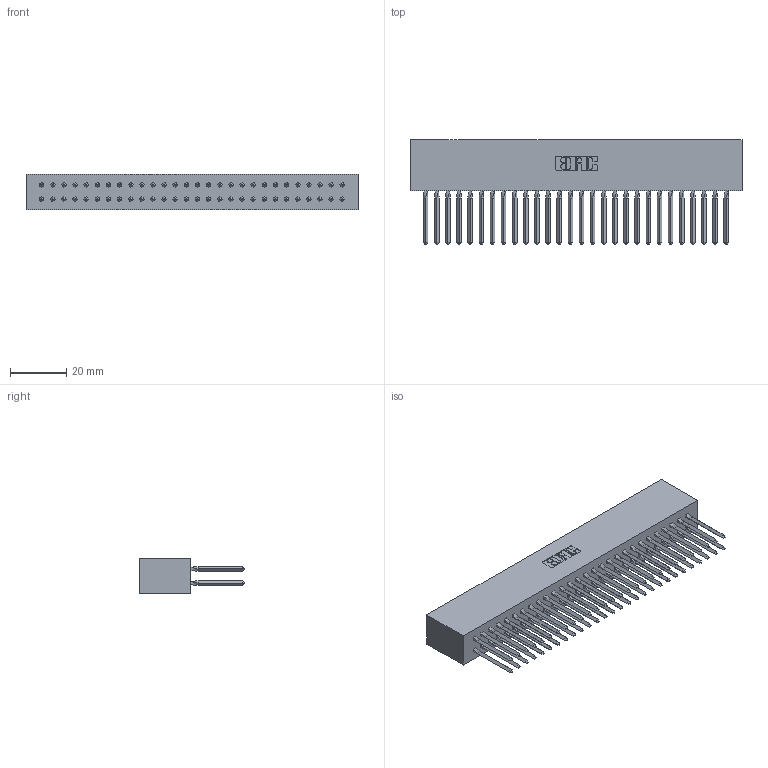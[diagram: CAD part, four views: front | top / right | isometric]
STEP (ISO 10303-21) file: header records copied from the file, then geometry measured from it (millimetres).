
FILE_DESCRIPTION (( 'STEP AP203' ), '1' );
FILE_NAME ('317-056-542-801.STEP', '2020-02-28T04:16:48', ( '' ), ( '' ), 'SwSTEP 2.0', 'SolidWorks 2016', '' );
FILE_SCHEMA (( 'CONFIG_CONTROL_DESIGN' ));
Length unit declared in the file: inch
Products named in the file (3): 317-290-003_542; 317-056-542-801; 317 Part_Lugless
Assembly tree (57 placements, depth 2):
  317-056-542-801
    317 Part_Lugless
    317-290-003_542  x56
Bounding box: 118.16 x 37.34 x 12.7 mm (x, y, z)
Volume: 20636.3 mm3; surface area: 28424.1 mm2
Topology: 57 solids, 57 shells, 3282 faces, 9199 edges, 5870 vertices
Faces by surface type: plane 2626, cylinder 432, bspline 224
Entity records: 41035 total; most frequent: CARTESIAN_POINT 7405, ORIENTED_EDGE 7068, DIRECTION 5962, EDGE_CURVE 3534, LINE 3372, VECTOR 3372, VERTEX_POINT 2350, AXIS2_PLACEMENT_3D 1295
